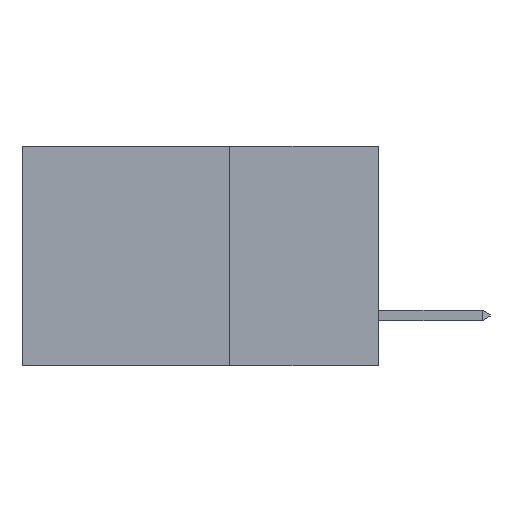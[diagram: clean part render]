
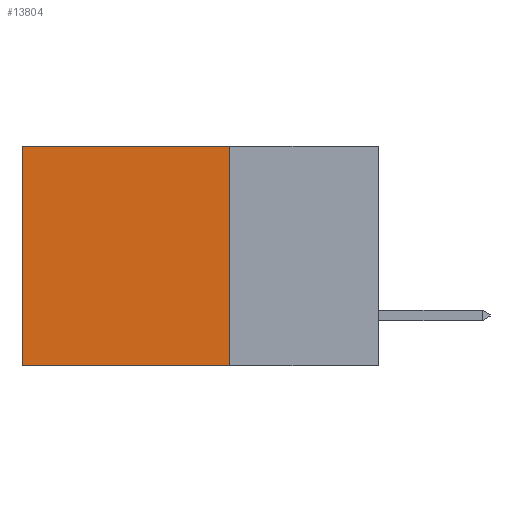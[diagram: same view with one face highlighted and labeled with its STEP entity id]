
A CAD part, left-side view. The second image highlights one B-rep face of the part: STEP entity #13804.
In plain terms, the highlighted planar face has unit normal (-1, 0, 0).
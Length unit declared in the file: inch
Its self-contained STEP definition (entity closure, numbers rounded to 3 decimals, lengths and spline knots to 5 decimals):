
#594 = DIRECTION ( 'NONE',  ( 0., 0., -1. ) ) ;
#1418 = ORIENTED_EDGE ( 'NONE', *, *, #10635, .F. ) ;
#1477 = EDGE_CURVE ( 'NONE', #9188, #10205, #5245, .T. ) ;
#1956 = CARTESIAN_POINT ( 'NONE',  ( 0.298, 0.6, -0.37 ) ) ;
#1986 = EDGE_CURVE ( 'NONE', #9188, #18902, #17024, .T. ) ;
#2557 = ORIENTED_EDGE ( 'NONE', *, *, #1986, .T. ) ;
#2970 = CARTESIAN_POINT ( 'NONE',  ( 0.298, 0.25, -0.37 ) ) ;
#3280 = CARTESIAN_POINT ( 'NONE',  ( 0.298, 0.6, 0. ) ) ;
#4158 = VECTOR ( 'NONE', #20175, 39.37008 ) ;
#4918 = DIRECTION ( 'NONE',  ( 0., 0., -1. ) ) ;
#5245 = LINE ( 'NONE', #19198, #17562 ) ;
#5783 = LINE ( 'NONE', #2970, #6288 ) ;
#5940 = VERTEX_POINT ( 'NONE', #1956 ) ;
#6256 = PLANE ( 'NONE',  #11481 ) ;
#6288 = VECTOR ( 'NONE', #9491, 39.37008 ) ;
#8397 = ORIENTED_EDGE ( 'NONE', *, *, #20792, .T. ) ;
#8824 = VECTOR ( 'NONE', #4918, 39.37008 ) ;
#9188 = VERTEX_POINT ( 'NONE', #17149 ) ;
#9491 = DIRECTION ( 'NONE',  ( 0., 1., 0. ) ) ;
#10205 = VERTEX_POINT ( 'NONE', #11602 ) ;
#10440 = EDGE_LOOP ( 'NONE', ( #8397, #1418, #13701, #2557 ) ) ;
#10635 = EDGE_CURVE ( 'NONE', #10205, #5940, #5783, .T. ) ;
#11165 = DIRECTION ( 'NONE',  ( 0., 0., -1. ) ) ;
#11481 = AXIS2_PLACEMENT_3D ( 'NONE', #15927, #20622, #11165 ) ;
#11602 = CARTESIAN_POINT ( 'NONE',  ( 0.298, 0.25, -0.37 ) ) ;
#13701 = ORIENTED_EDGE ( 'NONE', *, *, #1477, .F. ) ;
#13804 = ADVANCED_FACE ( 'NONE', ( #14718 ), #6256, .F. ) ;
#14718 = FACE_OUTER_BOUND ( 'NONE', #10440, .T. ) ;
#15305 = CARTESIAN_POINT ( 'NONE',  ( 0.298, 0.25, 0. ) ) ;
#15927 = CARTESIAN_POINT ( 'NONE',  ( 0.298, 0.25, 0. ) ) ;
#16370 = CARTESIAN_POINT ( 'NONE',  ( 0.298, 0.6, 0. ) ) ;
#17024 = LINE ( 'NONE', #15305, #4158 ) ;
#17149 = CARTESIAN_POINT ( 'NONE',  ( 0.298, 0.25, 0. ) ) ;
#17562 = VECTOR ( 'NONE', #594, 39.37008 ) ;
#17778 = LINE ( 'NONE', #3280, #8824 ) ;
#18902 = VERTEX_POINT ( 'NONE', #16370 ) ;
#19198 = CARTESIAN_POINT ( 'NONE',  ( 0.298, 0.25, 0. ) ) ;
#20175 = DIRECTION ( 'NONE',  ( 0., 1., 0. ) ) ;
#20622 = DIRECTION ( 'NONE',  ( 1., 0., 0. ) ) ;
#20792 = EDGE_CURVE ( 'NONE', #18902, #5940, #17778, .T. ) ;
